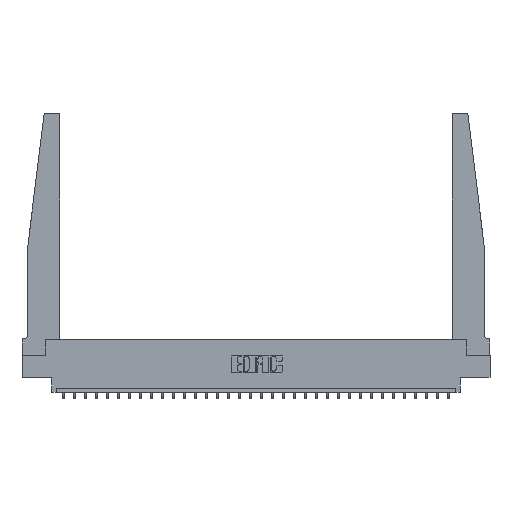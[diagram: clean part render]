
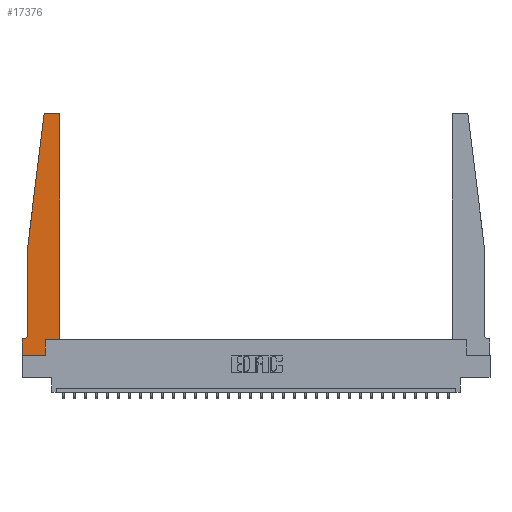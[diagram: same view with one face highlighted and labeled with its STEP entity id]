
A CAD part, top view. The second image highlights one B-rep face of the part: STEP entity #17376.
In plain terms, the highlighted planar face has unit normal (0, 0, 1).
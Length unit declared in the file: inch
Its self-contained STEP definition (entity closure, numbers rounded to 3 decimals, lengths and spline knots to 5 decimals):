
#54 = EDGE_CURVE ( 'NONE', #13150, #28393, #28486, .T. ) ;
#378 = CARTESIAN_POINT ( 'NONE',  ( 0.425, 0.18, 0.37 ) ) ;
#465 = DIRECTION ( 'NONE',  ( 0., 0., 1. ) ) ;
#520 = AXIS2_PLACEMENT_3D ( 'NONE', #22213, #2380, #25712 ) ;
#1619 = DIRECTION ( 'NONE',  ( -1., 0., 0. ) ) ;
#1779 = PLANE ( 'NONE',  #18738 ) ;
#1921 = CIRCLE ( 'NONE', #520, 0.03 ) ;
#2380 = DIRECTION ( 'NONE',  ( 0., 0., 1. ) ) ;
#2499 = CARTESIAN_POINT ( 'NONE',  ( 0.395, 2.72, 0.37 ) ) ;
#2540 = ORIENTED_EDGE ( 'NONE', *, *, #24802, .T. ) ;
#2633 = ORIENTED_EDGE ( 'NONE', *, *, #5499, .T. ) ;
#3261 = CARTESIAN_POINT ( 'NONE',  ( 0.425, 0.18, 0.37 ) ) ;
#3379 = VECTOR ( 'NONE', #16550, 39.37008 ) ;
#3394 = VECTOR ( 'NONE', #10603, 39.37008 ) ;
#3837 = VECTOR ( 'NONE', #14570, 39.37008 ) ;
#4131 = ORIENTED_EDGE ( 'NONE', *, *, #18597, .T. ) ;
#4402 = VERTEX_POINT ( 'NONE', #13236 ) ;
#4421 = CIRCLE ( 'NONE', #18231, 0.03 ) ;
#5184 = EDGE_CURVE ( 'NONE', #6328, #11364, #4421, .T. ) ;
#5499 = EDGE_CURVE ( 'NONE', #4402, #20320, #1921, .T. ) ;
#5585 = CARTESIAN_POINT ( 'NONE',  ( 0.425, 2.72, 0.37 ) ) ;
#6269 = DIRECTION ( 'NONE',  ( 1., 0., 0. ) ) ;
#6328 = VERTEX_POINT ( 'NONE', #5585 ) ;
#6529 = DIRECTION ( 'NONE',  ( 0., -1., 0. ) ) ;
#6692 = EDGE_LOOP ( 'NONE', ( #25798, #2633, #27936, #12576, #4131, #18869, #9963, #13770, #2540, #11487, #11097, #10260 ) ) ;
#7469 = EDGE_CURVE ( 'NONE', #11173, #12844, #20177, .T. ) ;
#7521 = CARTESIAN_POINT ( 'NONE',  ( 0.065, 1.25, 0.37 ) ) ;
#7706 = CARTESIAN_POINT ( 'NONE',  ( 0.065, 0.1875, 0.37 ) ) ;
#8030 = LINE ( 'NONE', #3261, #3837 ) ;
#8442 = DIRECTION ( 'NONE',  ( 0., 0., 1. ) ) ;
#8702 = VERTEX_POINT ( 'NONE', #21713 ) ;
#8720 = CARTESIAN_POINT ( 'NONE',  ( 0.065, 1.25, 0.37 ) ) ;
#8840 = CARTESIAN_POINT ( 'NONE',  ( 0., 0.1875, 0.37 ) ) ;
#9884 = LINE ( 'NONE', #7706, #3379 ) ;
#9963 = ORIENTED_EDGE ( 'NONE', *, *, #7469, .T. ) ;
#10146 = CARTESIAN_POINT ( 'NONE',  ( 0.25, 2.75, 0.37 ) ) ;
#10260 = ORIENTED_EDGE ( 'NONE', *, *, #5184, .T. ) ;
#10563 = LINE ( 'NONE', #10146, #13608 ) ;
#10576 = CARTESIAN_POINT ( 'NONE',  ( 0., 0.1875, 0.37 ) ) ;
#10603 = DIRECTION ( 'NONE',  ( 0., 1., 0. ) ) ;
#10990 = CARTESIAN_POINT ( 'NONE',  ( 0.425, 0.18, 0.37 ) ) ;
#11097 = ORIENTED_EDGE ( 'NONE', *, *, #26504, .T. ) ;
#11173 = VERTEX_POINT ( 'NONE', #8840 ) ;
#11364 = VERTEX_POINT ( 'NONE', #21372 ) ;
#11487 = ORIENTED_EDGE ( 'NONE', *, *, #13136, .T. ) ;
#12224 = VECTOR ( 'NONE', #13237, 39.37008 ) ;
#12417 = DIRECTION ( 'NONE',  ( 1., 0., 0. ) ) ;
#12576 = ORIENTED_EDGE ( 'NONE', *, *, #54, .T. ) ;
#12717 = VECTOR ( 'NONE', #24304, 39.37008 ) ;
#12844 = VERTEX_POINT ( 'NONE', #19776 ) ;
#13038 = VERTEX_POINT ( 'NONE', #378 ) ;
#13136 = EDGE_CURVE ( 'NONE', #19360, #13038, #8030, .T. ) ;
#13142 = DIRECTION ( 'NONE',  ( -1., 0., 0. ) ) ;
#13150 = VERTEX_POINT ( 'NONE', #23363 ) ;
#13236 = CARTESIAN_POINT ( 'NONE',  ( 0.27653, 2.75, 0.37 ) ) ;
#13237 = DIRECTION ( 'NONE',  ( 0., -1., 0. ) ) ;
#13350 = CARTESIAN_POINT ( 'NONE',  ( 0.2605, 0.18, 0.37 ) ) ;
#13530 = EDGE_CURVE ( 'NONE', #8702, #11173, #9884, .T. ) ;
#13608 = VECTOR ( 'NONE', #1619, 39.37008 ) ;
#13770 = ORIENTED_EDGE ( 'NONE', *, *, #27775, .T. ) ;
#14570 = DIRECTION ( 'NONE',  ( 1., 0., 0. ) ) ;
#14788 = LINE ( 'NONE', #23429, #21046 ) ;
#15503 = LINE ( 'NONE', #10990, #12717 ) ;
#15544 = AXIS2_PLACEMENT_3D ( 'NONE', #22548, #27008, #13142 ) ;
#15545 = CARTESIAN_POINT ( 'NONE',  ( 0.2605, 0.18, 0.37 ) ) ;
#16150 = EDGE_CURVE ( 'NONE', #20320, #13150, #20669, .T. ) ;
#16550 = DIRECTION ( 'NONE',  ( -1., 0., 0. ) ) ;
#16967 = CARTESIAN_POINT ( 'NONE',  ( 0.065, 0.2375, 0.37 ) ) ;
#17376 = ADVANCED_FACE ( 'NONE', ( #21589 ), #1779, .T. ) ;
#17389 = CIRCLE ( 'NONE', #15544, 0.05 ) ;
#17508 = VECTOR ( 'NONE', #6529, 39.37008 ) ;
#18231 = AXIS2_PLACEMENT_3D ( 'NONE', #2499, #465, #26346 ) ;
#18400 = CARTESIAN_POINT ( 'NONE',  ( 0.24675, 2.72367, 0.37 ) ) ;
#18597 = EDGE_CURVE ( 'NONE', #28393, #8702, #17389, .T. ) ;
#18738 = AXIS2_PLACEMENT_3D ( 'NONE', #10576, #8442, #6269 ) ;
#18869 = ORIENTED_EDGE ( 'NONE', *, *, #13530, .T. ) ;
#19360 = VERTEX_POINT ( 'NONE', #15545 ) ;
#19653 = VECTOR ( 'NONE', #20807, 39.37008 ) ;
#19776 = CARTESIAN_POINT ( 'NONE',  ( 0., 0., 0.37 ) ) ;
#20177 = LINE ( 'NONE', #26235, #12224 ) ;
#20320 = VERTEX_POINT ( 'NONE', #18400 ) ;
#20669 = LINE ( 'NONE', #7521, #19653 ) ;
#20807 = DIRECTION ( 'NONE',  ( -0.122, -0.992, 0. ) ) ;
#21046 = VECTOR ( 'NONE', #12417, 39.37008 ) ;
#21372 = CARTESIAN_POINT ( 'NONE',  ( 0.395, 2.75, 0.37 ) ) ;
#21589 = FACE_OUTER_BOUND ( 'NONE', #6692, .T. ) ;
#21713 = CARTESIAN_POINT ( 'NONE',  ( 0.015, 0.1875, 0.37 ) ) ;
#21767 = CARTESIAN_POINT ( 'NONE',  ( 0.2605, 0., 0.37 ) ) ;
#22213 = CARTESIAN_POINT ( 'NONE',  ( 0.27653, 2.72, 0.37 ) ) ;
#22548 = CARTESIAN_POINT ( 'NONE',  ( 0.015, 0.2375, 0.37 ) ) ;
#23363 = CARTESIAN_POINT ( 'NONE',  ( 0.065, 1.25, 0.37 ) ) ;
#23429 = CARTESIAN_POINT ( 'NONE',  ( 0., 0., 0.37 ) ) ;
#24304 = DIRECTION ( 'NONE',  ( 0., 1., 0. ) ) ;
#24345 = LINE ( 'NONE', #13350, #3394 ) ;
#24802 = EDGE_CURVE ( 'NONE', #27544, #19360, #24345, .T. ) ;
#25712 = DIRECTION ( 'NONE',  ( 1., 0., 0. ) ) ;
#25798 = ORIENTED_EDGE ( 'NONE', *, *, #26063, .T. ) ;
#26063 = EDGE_CURVE ( 'NONE', #11364, #4402, #10563, .T. ) ;
#26235 = CARTESIAN_POINT ( 'NONE',  ( 0., 0., 0.37 ) ) ;
#26346 = DIRECTION ( 'NONE',  ( 1., 0., 0. ) ) ;
#26504 = EDGE_CURVE ( 'NONE', #13038, #6328, #15503, .T. ) ;
#27008 = DIRECTION ( 'NONE',  ( 0., 0., -1. ) ) ;
#27544 = VERTEX_POINT ( 'NONE', #21767 ) ;
#27775 = EDGE_CURVE ( 'NONE', #12844, #27544, #14788, .T. ) ;
#27936 = ORIENTED_EDGE ( 'NONE', *, *, #16150, .T. ) ;
#28393 = VERTEX_POINT ( 'NONE', #16967 ) ;
#28486 = LINE ( 'NONE', #8720, #17508 ) ;
